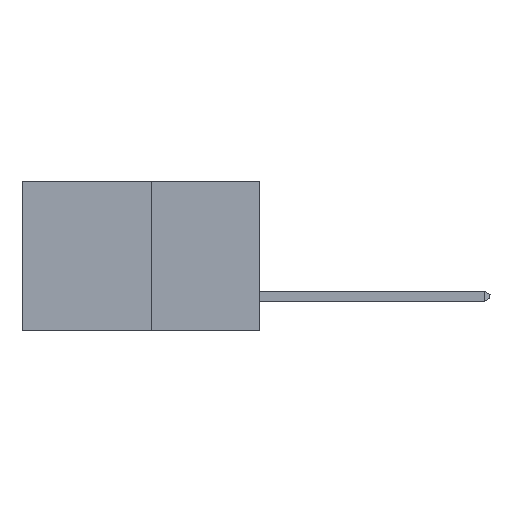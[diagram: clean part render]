
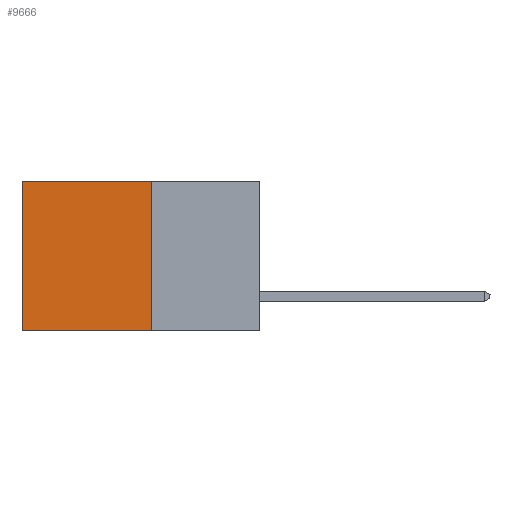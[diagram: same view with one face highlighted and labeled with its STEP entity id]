
A CAD part, left-side view. The second image highlights one B-rep face of the part: STEP entity #9666.
In plain terms, the highlighted planar face has unit normal (-1, 0, 0).
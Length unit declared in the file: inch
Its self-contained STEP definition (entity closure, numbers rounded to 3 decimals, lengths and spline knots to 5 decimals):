
#353 = DIRECTION ( 'NONE',  ( 0., 0., -1. ) ) ;
#403 = ORIENTED_EDGE ( 'NONE', *, *, #3718, .F. ) ;
#473 = LINE ( 'NONE', #9991, #5276 ) ;
#553 = CARTESIAN_POINT ( 'NONE',  ( 0.277, 0.59, -0.37 ) ) ;
#676 = VERTEX_POINT ( 'NONE', #11904 ) ;
#1160 = DIRECTION ( 'NONE',  ( 0., 1., 0. ) ) ;
#1208 = CARTESIAN_POINT ( 'NONE',  ( 0.277, 0.27, 0. ) ) ;
#2369 = VERTEX_POINT ( 'NONE', #2674 ) ;
#2496 = VECTOR ( 'NONE', #7386, 39.37008 ) ;
#2674 = CARTESIAN_POINT ( 'NONE',  ( 0.277, 0.59, 0. ) ) ;
#3718 = EDGE_CURVE ( 'NONE', #4176, #676, #7730, .T. ) ;
#4018 = EDGE_LOOP ( 'NONE', ( #6478, #403, #6630, #4796 ) ) ;
#4069 = VERTEX_POINT ( 'NONE', #10308 ) ;
#4130 = LINE ( 'NONE', #553, #8680 ) ;
#4176 = VERTEX_POINT ( 'NONE', #8768 ) ;
#4418 = PLANE ( 'NONE',  #11597 ) ;
#4564 = VECTOR ( 'NONE', #1160, 39.37008 ) ;
#4796 = ORIENTED_EDGE ( 'NONE', *, *, #6896, .T. ) ;
#5000 = EDGE_CURVE ( 'NONE', #4069, #4176, #473, .T. ) ;
#5276 = VECTOR ( 'NONE', #10009, 39.37008 ) ;
#5330 = DIRECTION ( 'NONE',  ( 0., 0., -1. ) ) ;
#6478 = ORIENTED_EDGE ( 'NONE', *, *, #6968, .T. ) ;
#6630 = ORIENTED_EDGE ( 'NONE', *, *, #5000, .F. ) ;
#6896 = EDGE_CURVE ( 'NONE', #4069, #2369, #7269, .T. ) ;
#6968 = EDGE_CURVE ( 'NONE', #2369, #676, #4130, .T. ) ;
#7269 = LINE ( 'NONE', #1208, #4564 ) ;
#7386 = DIRECTION ( 'NONE',  ( 0., 1., 0. ) ) ;
#7521 = FACE_OUTER_BOUND ( 'NONE', #4018, .T. ) ;
#7700 = CARTESIAN_POINT ( 'NONE',  ( 0.277, 0.27, -0.37 ) ) ;
#7730 = LINE ( 'NONE', #7700, #2496 ) ;
#8025 = CARTESIAN_POINT ( 'NONE',  ( 0.277, 0.27, -0.37 ) ) ;
#8680 = VECTOR ( 'NONE', #353, 39.37008 ) ;
#8768 = CARTESIAN_POINT ( 'NONE',  ( 0.277, 0.27, -0.37 ) ) ;
#9666 = ADVANCED_FACE ( 'NONE', ( #7521 ), #4418, .F. ) ;
#9991 = CARTESIAN_POINT ( 'NONE',  ( 0.277, 0.27, -0.37 ) ) ;
#10009 = DIRECTION ( 'NONE',  ( 0., 0., -1. ) ) ;
#10308 = CARTESIAN_POINT ( 'NONE',  ( 0.277, 0.27, 0. ) ) ;
#10693 = DIRECTION ( 'NONE',  ( 1., 0., 0. ) ) ;
#11597 = AXIS2_PLACEMENT_3D ( 'NONE', #8025, #10693, #5330 ) ;
#11904 = CARTESIAN_POINT ( 'NONE',  ( 0.277, 0.59, -0.37 ) ) ;
